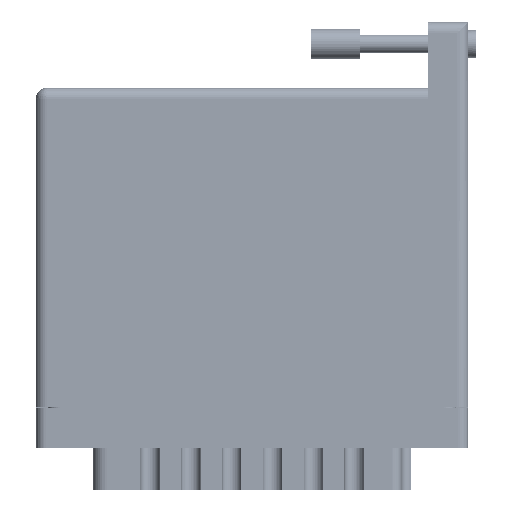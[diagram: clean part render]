
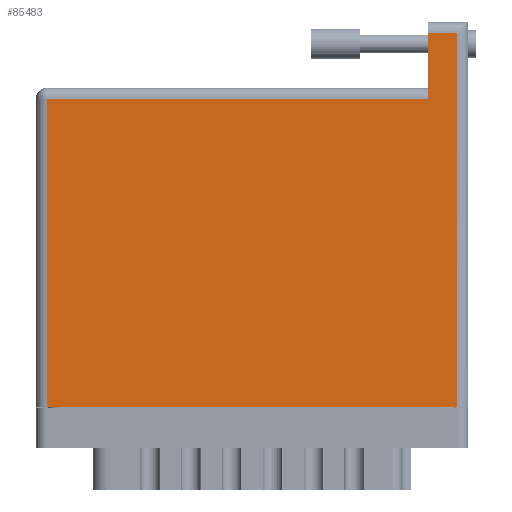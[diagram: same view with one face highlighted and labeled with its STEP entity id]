
A CAD part, front view. The second image highlights one B-rep face of the part: STEP entity #85483.
In plain terms, the highlighted face is planar.
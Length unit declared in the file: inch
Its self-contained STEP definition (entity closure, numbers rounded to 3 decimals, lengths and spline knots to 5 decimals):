
#295 = VECTOR ( 'NONE', #77485, 39.37008 ) ;
#346 = VECTOR ( 'NONE', #36864, 39.37008 ) ;
#623 = CARTESIAN_POINT ( 'NONE',  ( 2.499, 1.96, 0. ) ) ;
#1789 = CARTESIAN_POINT ( 'NONE',  ( 0., 1.96, 0. ) ) ;
#4640 = EDGE_CURVE ( 'NONE', #33015, #53684, #62181, .T. ) ;
#5619 = CARTESIAN_POINT ( 'NONE',  ( 2.499, 2.45, 0. ) ) ;
#5808 = DIRECTION ( 'NONE',  ( -1., 0., 0. ) ) ;
#9151 = FACE_OUTER_BOUND ( 'NONE', #57125, .T. ) ;
#10909 = ORIENTED_EDGE ( 'NONE', *, *, #48478, .T. ) ;
#11541 = CARTESIAN_POINT ( 'NONE',  ( 0.07, 0., 0. ) ) ;
#11998 = DIRECTION ( 'NONE',  ( 0., 1., 0. ) ) ;
#13369 = VECTOR ( 'NONE', #5808, 39.37008 ) ;
#18412 = EDGE_CURVE ( 'NONE', #57813, #33015, #92781, .T. ) ;
#20230 = AXIS2_PLACEMENT_3D ( 'NONE', #52795, #81476, #66456 ) ;
#21374 = CARTESIAN_POINT ( 'NONE',  ( 0.07, 0., 0. ) ) ;
#24146 = PLANE ( 'NONE',  #20230 ) ;
#25703 = CARTESIAN_POINT ( 'NONE',  ( 2.499, 2.38, 0. ) ) ;
#30462 = DIRECTION ( 'NONE',  ( -1., 0., 0. ) ) ;
#33015 = VERTEX_POINT ( 'NONE', #11541 ) ;
#33692 = VERTEX_POINT ( 'NONE', #63078 ) ;
#34540 = LINE ( 'NONE', #75454, #41161 ) ;
#36864 = DIRECTION ( 'NONE',  ( 0., -1., 0. ) ) ;
#40569 = CARTESIAN_POINT ( 'NONE',  ( 0., 0., 0. ) ) ;
#41161 = VECTOR ( 'NONE', #11998, 39.37008 ) ;
#42017 = ORIENTED_EDGE ( 'NONE', *, *, #70120, .T. ) ;
#44217 = ORIENTED_EDGE ( 'NONE', *, *, #18412, .T. ) ;
#45899 = LINE ( 'NONE', #77684, #13369 ) ;
#48478 = EDGE_CURVE ( 'NONE', #91792, #57813, #66137, .T. ) ;
#49280 = ORIENTED_EDGE ( 'NONE', *, *, #4640, .T. ) ;
#52795 = CARTESIAN_POINT ( 'NONE',  ( 0., 2.03, 0. ) ) ;
#53684 = VERTEX_POINT ( 'NONE', #74684 ) ;
#54131 = CARTESIAN_POINT ( 'NONE',  ( 0.07, 1.96, 0. ) ) ;
#57125 = EDGE_LOOP ( 'NONE', ( #76674, #10909, #44217, #49280, #42017, #91921 ) ) ;
#57813 = VERTEX_POINT ( 'NONE', #54131 ) ;
#62028 = VERTEX_POINT ( 'NONE', #25703 ) ;
#62181 = LINE ( 'NONE', #40569, #88761 ) ;
#63078 = CARTESIAN_POINT ( 'NONE',  ( 2.685, 2.38, 0. ) ) ;
#66137 = LINE ( 'NONE', #1789, #75220 ) ;
#66456 = DIRECTION ( 'NONE',  ( -1., 0., 0. ) ) ;
#69495 = LINE ( 'NONE', #5619, #295 ) ;
#70120 = EDGE_CURVE ( 'NONE', #53684, #33692, #34540, .T. ) ;
#74684 = CARTESIAN_POINT ( 'NONE',  ( 2.685, 0., 0. ) ) ;
#74901 = EDGE_CURVE ( 'NONE', #62028, #91792, #69495, .T. ) ;
#75220 = VECTOR ( 'NONE', #30462, 39.37008 ) ;
#75454 = CARTESIAN_POINT ( 'NONE',  ( 2.685, 2.45, 0. ) ) ;
#76674 = ORIENTED_EDGE ( 'NONE', *, *, #74901, .T. ) ;
#77485 = DIRECTION ( 'NONE',  ( 0., -1., 0. ) ) ;
#77684 = CARTESIAN_POINT ( 'NONE',  ( 0., 2.38, 0. ) ) ;
#81476 = DIRECTION ( 'NONE',  ( 0., 0., -1. ) ) ;
#83784 = DIRECTION ( 'NONE',  ( 1., 0., 0. ) ) ;
#85483 = ADVANCED_FACE ( 'NONE', ( #9151 ), #24146, .F. ) ;
#88761 = VECTOR ( 'NONE', #83784, 39.37008 ) ;
#91611 = EDGE_CURVE ( 'NONE', #33692, #62028, #45899, .T. ) ;
#91792 = VERTEX_POINT ( 'NONE', #623 ) ;
#91921 = ORIENTED_EDGE ( 'NONE', *, *, #91611, .T. ) ;
#92781 = LINE ( 'NONE', #21374, #346 ) ;
